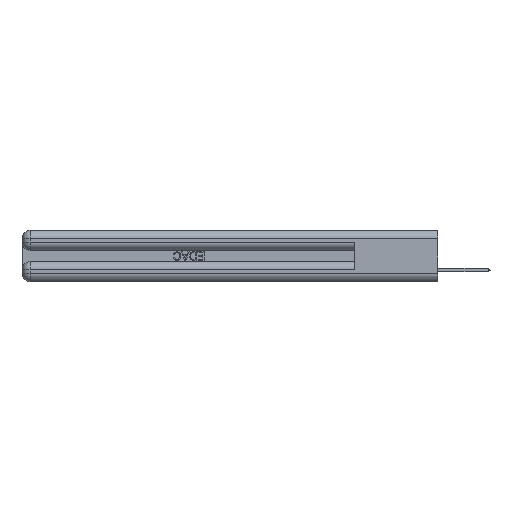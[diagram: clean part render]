
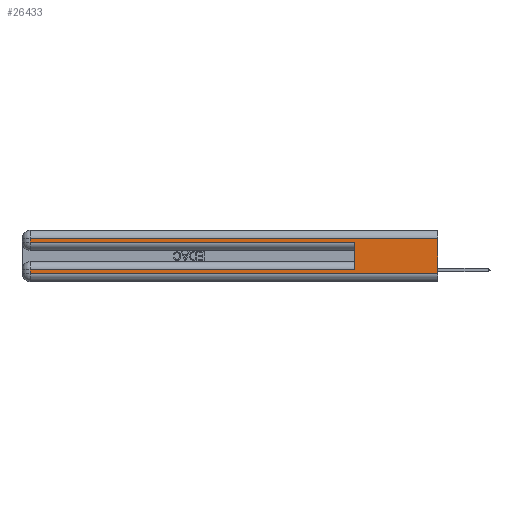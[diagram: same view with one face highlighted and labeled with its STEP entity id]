
A CAD part, left-side view. The second image highlights one B-rep face of the part: STEP entity #26433.
In plain terms, the highlighted planar face has unit normal (-1, 0, 0).
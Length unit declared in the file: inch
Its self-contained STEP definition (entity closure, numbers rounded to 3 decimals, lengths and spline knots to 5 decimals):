
#359 = ORIENTED_EDGE ( 'NONE', *, *, #21661, .T. ) ;
#584 = VECTOR ( 'NONE', #15085, 39.37008 ) ;
#806 = VECTOR ( 'NONE', #36116, 39.37008 ) ;
#1150 = CARTESIAN_POINT ( 'NONE',  ( 0., 0., 0.31 ) ) ;
#1610 = CARTESIAN_POINT ( 'NONE',  ( 0., 2.94, 0.37 ) ) ;
#1713 = CARTESIAN_POINT ( 'NONE',  ( 0., 0., 0.37 ) ) ;
#1910 = LINE ( 'NONE', #26660, #806 ) ;
#2870 = VERTEX_POINT ( 'NONE', #3767 ) ;
#3767 = CARTESIAN_POINT ( 'NONE',  ( 0., 0.6, 0.285 ) ) ;
#4477 = LINE ( 'NONE', #11334, #42364 ) ;
#4555 = EDGE_CURVE ( 'NONE', #19382, #38289, #1910, .T. ) ;
#6328 = LINE ( 'NONE', #31321, #584 ) ;
#7556 = LINE ( 'NONE', #19371, #27499 ) ;
#8437 = DIRECTION ( 'NONE',  ( 0., 0., -1. ) ) ;
#9572 = VECTOR ( 'NONE', #8437, 39.37008 ) ;
#10363 = CARTESIAN_POINT ( 'NONE',  ( 0., 2.94, 0.31 ) ) ;
#10813 = ORIENTED_EDGE ( 'NONE', *, *, #36655, .T. ) ;
#11156 = CARTESIAN_POINT ( 'NONE',  ( 0., 0., 0.06 ) ) ;
#11334 = CARTESIAN_POINT ( 'NONE',  ( 0., 0., 0.31 ) ) ;
#12056 = CARTESIAN_POINT ( 'NONE',  ( 0., 0., 0.37 ) ) ;
#14562 = VERTEX_POINT ( 'NONE', #1150 ) ;
#15085 = DIRECTION ( 'NONE',  ( 0., 0., 1. ) ) ;
#15168 = DIRECTION ( 'NONE',  ( 0., -1., 0. ) ) ;
#15592 = CARTESIAN_POINT ( 'NONE',  ( 0., 2.94, 0.06 ) ) ;
#17034 = ORIENTED_EDGE ( 'NONE', *, *, #4555, .T. ) ;
#17356 = EDGE_CURVE ( 'NONE', #14562, #19382, #4477, .T. ) ;
#17878 = CARTESIAN_POINT ( 'NONE',  ( 0., 0., 0.06 ) ) ;
#17899 = DIRECTION ( 'NONE',  ( 0., 1., 0. ) ) ;
#18460 = EDGE_CURVE ( 'NONE', #14562, #41807, #30444, .T. ) ;
#18494 = VERTEX_POINT ( 'NONE', #15592 ) ;
#18931 = DIRECTION ( 'NONE',  ( 0., 0., -1. ) ) ;
#19371 = CARTESIAN_POINT ( 'NONE',  ( 0., 0., 0.285 ) ) ;
#19382 = VERTEX_POINT ( 'NONE', #10363 ) ;
#19407 = VERTEX_POINT ( 'NONE', #37357 ) ;
#21661 = EDGE_CURVE ( 'NONE', #19407, #38591, #37500, .T. ) ;
#23636 = CARTESIAN_POINT ( 'NONE',  ( 0., 2.94, 0.285 ) ) ;
#24139 = AXIS2_PLACEMENT_3D ( 'NONE', #1713, #28486, #18931 ) ;
#25517 = VECTOR ( 'NONE', #15168, 39.37008 ) ;
#26433 = ADVANCED_FACE ( 'NONE', ( #41410 ), #37186, .F. ) ;
#26660 = CARTESIAN_POINT ( 'NONE',  ( 0., 2.94, 0.37 ) ) ;
#27186 = ORIENTED_EDGE ( 'NONE', *, *, #17356, .T. ) ;
#27465 = ORIENTED_EDGE ( 'NONE', *, *, #29985, .T. ) ;
#27499 = VECTOR ( 'NONE', #37079, 39.37008 ) ;
#28486 = DIRECTION ( 'NONE',  ( 1., 0., 0. ) ) ;
#29686 = EDGE_CURVE ( 'NONE', #38289, #2870, #7556, .T. ) ;
#29985 = EDGE_CURVE ( 'NONE', #38591, #18494, #35183, .T. ) ;
#30444 = LINE ( 'NONE', #12056, #9572 ) ;
#31321 = CARTESIAN_POINT ( 'NONE',  ( 0., 0.6, 0.145 ) ) ;
#31422 = EDGE_LOOP ( 'NONE', ( #40973, #27186, #17034, #32122, #33162, #359, #27465, #10813 ) ) ;
#32122 = ORIENTED_EDGE ( 'NONE', *, *, #29686, .T. ) ;
#33162 = ORIENTED_EDGE ( 'NONE', *, *, #39955, .F. ) ;
#33553 = VECTOR ( 'NONE', #37495, 39.37008 ) ;
#34150 = LINE ( 'NONE', #17878, #25517 ) ;
#35183 = LINE ( 'NONE', #1610, #33553 ) ;
#35465 = CARTESIAN_POINT ( 'NONE',  ( 0., 0., 0.085 ) ) ;
#36116 = DIRECTION ( 'NONE',  ( 0., 0., -1. ) ) ;
#36655 = EDGE_CURVE ( 'NONE', #18494, #41807, #34150, .T. ) ;
#37079 = DIRECTION ( 'NONE',  ( 0., -1., 0. ) ) ;
#37186 = PLANE ( 'NONE',  #24139 ) ;
#37357 = CARTESIAN_POINT ( 'NONE',  ( 0., 0.6, 0.085 ) ) ;
#37495 = DIRECTION ( 'NONE',  ( 0., 0., -1. ) ) ;
#37500 = LINE ( 'NONE', #35465, #41630 ) ;
#38114 = CARTESIAN_POINT ( 'NONE',  ( 0., 2.94, 0.085 ) ) ;
#38289 = VERTEX_POINT ( 'NONE', #23636 ) ;
#38591 = VERTEX_POINT ( 'NONE', #38114 ) ;
#39760 = DIRECTION ( 'NONE',  ( 0., 1., 0. ) ) ;
#39955 = EDGE_CURVE ( 'NONE', #19407, #2870, #6328, .T. ) ;
#40973 = ORIENTED_EDGE ( 'NONE', *, *, #18460, .F. ) ;
#41410 = FACE_OUTER_BOUND ( 'NONE', #31422, .T. ) ;
#41630 = VECTOR ( 'NONE', #17899, 39.37008 ) ;
#41807 = VERTEX_POINT ( 'NONE', #11156 ) ;
#42364 = VECTOR ( 'NONE', #39760, 39.37008 ) ;
